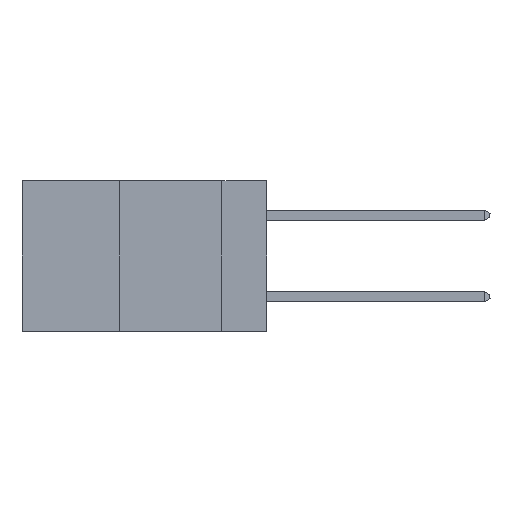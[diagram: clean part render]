
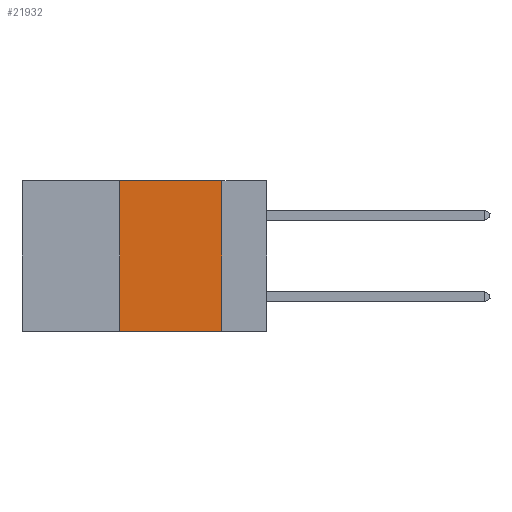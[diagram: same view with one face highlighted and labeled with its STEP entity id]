
A CAD part, left-side view. The second image highlights one B-rep face of the part: STEP entity #21932.
In plain terms, the highlighted planar face has unit normal (-1, 0, 0).
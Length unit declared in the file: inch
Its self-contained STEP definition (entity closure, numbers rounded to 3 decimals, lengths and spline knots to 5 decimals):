
#732 = EDGE_LOOP ( 'NONE', ( #22305, #19154, #9474, #22710 ) ) ;
#927 = EDGE_CURVE ( 'NONE', #17356, #6311, #21904, .T. ) ;
#2829 = VECTOR ( 'NONE', #7319, 39.37008 ) ;
#3710 = EDGE_CURVE ( 'NONE', #6734, #6311, #6739, .T. ) ;
#5112 = CARTESIAN_POINT ( 'NONE',  ( 0., 0.6, 0. ) ) ;
#5325 = CARTESIAN_POINT ( 'NONE',  ( 0., 0.11, 0. ) ) ;
#5571 = DIRECTION ( 'NONE',  ( 0., 0., -1. ) ) ;
#5573 = VECTOR ( 'NONE', #23453, 39.37008 ) ;
#6311 = VERTEX_POINT ( 'NONE', #16991 ) ;
#6734 = VERTEX_POINT ( 'NONE', #12625 ) ;
#6739 = LINE ( 'NONE', #5325, #15386 ) ;
#7064 = DIRECTION ( 'NONE',  ( 0., 0., -1. ) ) ;
#7235 = CARTESIAN_POINT ( 'NONE',  ( 0., 0.36, 0. ) ) ;
#7319 = DIRECTION ( 'NONE',  ( 0., -1., 0. ) ) ;
#7891 = LINE ( 'NONE', #21561, #17063 ) ;
#8640 = CARTESIAN_POINT ( 'NONE',  ( 0., 0.6, -0.37 ) ) ;
#8652 = EDGE_CURVE ( 'NONE', #19198, #6734, #15444, .T. ) ;
#9474 = ORIENTED_EDGE ( 'NONE', *, *, #23928, .F. ) ;
#12625 = CARTESIAN_POINT ( 'NONE',  ( 0., 0.11, 0. ) ) ;
#14319 = PLANE ( 'NONE',  #15133 ) ;
#15133 = AXIS2_PLACEMENT_3D ( 'NONE', #5112, #18067, #7064 ) ;
#15386 = VECTOR ( 'NONE', #5571, 39.37008 ) ;
#15444 = LINE ( 'NONE', #21621, #5573 ) ;
#16991 = CARTESIAN_POINT ( 'NONE',  ( 0., 0.11, -0.37 ) ) ;
#17063 = VECTOR ( 'NONE', #23397, 39.37008 ) ;
#17356 = VERTEX_POINT ( 'NONE', #19680 ) ;
#18067 = DIRECTION ( 'NONE',  ( 1., 0., 0. ) ) ;
#19154 = ORIENTED_EDGE ( 'NONE', *, *, #8652, .F. ) ;
#19198 = VERTEX_POINT ( 'NONE', #7235 ) ;
#19680 = CARTESIAN_POINT ( 'NONE',  ( 0., 0.36, -0.37 ) ) ;
#21561 = CARTESIAN_POINT ( 'NONE',  ( 0., 0.36, 0. ) ) ;
#21621 = CARTESIAN_POINT ( 'NONE',  ( 0., 0.6, 0. ) ) ;
#21904 = LINE ( 'NONE', #8640, #2829 ) ;
#21932 = ADVANCED_FACE ( 'NONE', ( #23628 ), #14319, .F. ) ;
#22305 = ORIENTED_EDGE ( 'NONE', *, *, #3710, .F. ) ;
#22710 = ORIENTED_EDGE ( 'NONE', *, *, #927, .T. ) ;
#23397 = DIRECTION ( 'NONE',  ( 0., 0., 1. ) ) ;
#23453 = DIRECTION ( 'NONE',  ( 0., -1., 0. ) ) ;
#23628 = FACE_OUTER_BOUND ( 'NONE', #732, .T. ) ;
#23928 = EDGE_CURVE ( 'NONE', #17356, #19198, #7891, .T. ) ;
